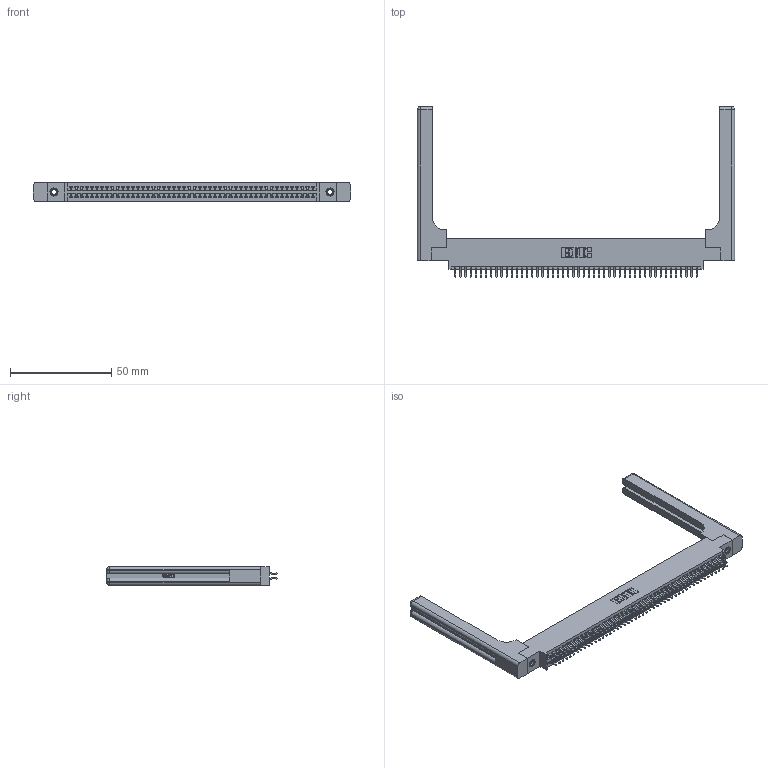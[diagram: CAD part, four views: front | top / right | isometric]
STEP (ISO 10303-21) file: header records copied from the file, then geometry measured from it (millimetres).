
FILE_DESCRIPTION (( 'STEP AP203' ), '1' );
FILE_NAME ('345-096-556-858.STEP', '2019-11-02T09:04:38', ( '' ), ( '' ), 'SwSTEP 2.0', 'SolidWorks 2016', '' );
FILE_SCHEMA (( 'CONFIG_CONTROL_DESIGN' ));
Length unit declared in the file: inch
Products named in the file (5): 345-250-001_345-250-001-102; 345-292-001_556 Tail; 345-096-556-858; 345-220-058_345-220-058; 345 Part_0.170 Offset - 0.156 Dia-TH
Assembly tree (101 placements, depth 2):
  345-096-556-858
    345 Part_0.170 Offset - 0.156 Dia-TH
    345-292-001_556 Tail  x96
    345-250-001_345-250-001-102  x2
    345-220-058_345-220-058  x2
Bounding box: 156.95 x 84.51 x 9.4 mm (x, y, z)
Volume: 23659.6 mm3; surface area: 27679.7 mm2
Topology: 101 solids, 101 shells, 5762 faces, 17051 edges, 11218 vertices
Faces by surface type: plane 3784, cylinder 1918, bspline 36, cone 12, sphere 8, torus 4
Entity records: 42388 total; most frequent: CARTESIAN_POINT 8109, ORIENTED_EDGE 6828, DIRECTION 6062, EDGE_CURVE 3414, VECTOR 2990, LINE 2990, VERTEX_POINT 2266, AXIS2_PLACEMENT_3D 1536
